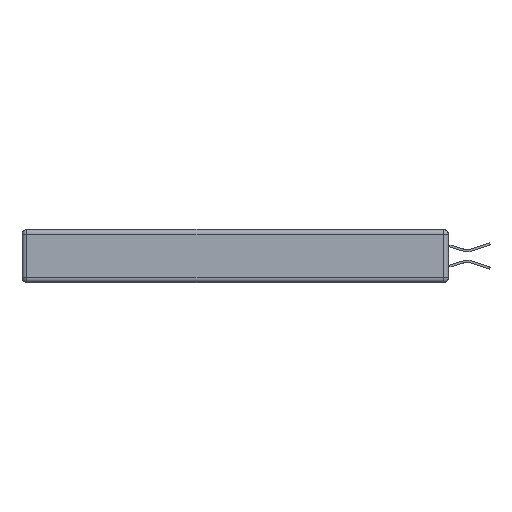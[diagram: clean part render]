
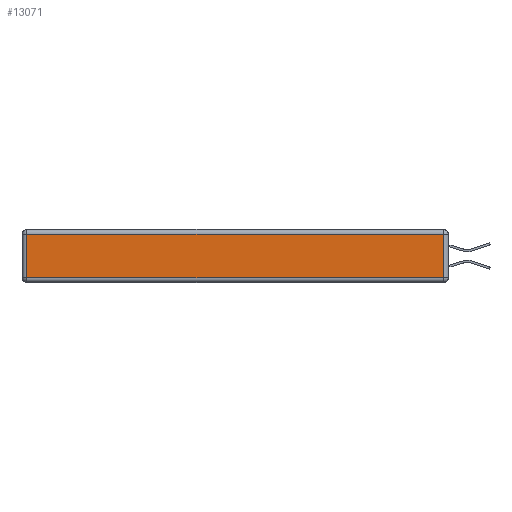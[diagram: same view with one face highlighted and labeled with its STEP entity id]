
A CAD part, left-side view. The second image highlights one B-rep face of the part: STEP entity #13071.
In plain terms, the highlighted planar face has unit normal (-1, 0, 0).
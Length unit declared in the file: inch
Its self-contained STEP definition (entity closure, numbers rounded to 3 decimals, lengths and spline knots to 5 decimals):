
#845 = CARTESIAN_POINT ( 'NONE',  ( 0., 2.72, -0.313 ) ) ;
#970 = VERTEX_POINT ( 'NONE', #845 ) ;
#1485 = EDGE_LOOP ( 'NONE', ( #31062, #12189, #10361, #12286 ) ) ;
#4456 = LINE ( 'NONE', #27313, #30382 ) ;
#4664 = CARTESIAN_POINT ( 'NONE',  ( 0., 0.03, -0.343 ) ) ;
#5438 = CARTESIAN_POINT ( 'NONE',  ( 0., 2.75, -0.03 ) ) ;
#6064 = LINE ( 'NONE', #5438, #15171 ) ;
#7155 = PLANE ( 'NONE',  #19806 ) ;
#8004 = DIRECTION ( 'NONE',  ( 0., 1., 0. ) ) ;
#8009 = CARTESIAN_POINT ( 'NONE',  ( 0., 0.03, -0.313 ) ) ;
#10361 = ORIENTED_EDGE ( 'NONE', *, *, #16900, .T. ) ;
#12189 = ORIENTED_EDGE ( 'NONE', *, *, #26618, .T. ) ;
#12286 = ORIENTED_EDGE ( 'NONE', *, *, #23566, .T. ) ;
#13071 = ADVANCED_FACE ( 'NONE', ( #21652 ), #7155, .T. ) ;
#14498 = VERTEX_POINT ( 'NONE', #23048 ) ;
#15023 = VERTEX_POINT ( 'NONE', #27066 ) ;
#15171 = VECTOR ( 'NONE', #8004, 39.37008 ) ;
#16363 = DIRECTION ( 'NONE',  ( 0., 0., 1. ) ) ;
#16900 = EDGE_CURVE ( 'NONE', #15023, #14498, #6064, .T. ) ;
#19366 = DIRECTION ( 'NONE',  ( -1., 0., 0. ) ) ;
#19806 = AXIS2_PLACEMENT_3D ( 'NONE', #31327, #19366, #24188 ) ;
#21652 = FACE_OUTER_BOUND ( 'NONE', #1485, .T. ) ;
#21655 = CARTESIAN_POINT ( 'NONE',  ( 0., 2.72, -0.343 ) ) ;
#22285 = DIRECTION ( 'NONE',  ( 0., -1., 0. ) ) ;
#23048 = CARTESIAN_POINT ( 'NONE',  ( 0., 2.72, -0.03 ) ) ;
#23566 = EDGE_CURVE ( 'NONE', #14498, #970, #24446, .T. ) ;
#24188 = DIRECTION ( 'NONE',  ( 0., 0., 1. ) ) ;
#24446 = LINE ( 'NONE', #21655, #29399 ) ;
#25673 = EDGE_CURVE ( 'NONE', #970, #28129, #4456, .T. ) ;
#26451 = DIRECTION ( 'NONE',  ( 0., 0., -1. ) ) ;
#26618 = EDGE_CURVE ( 'NONE', #28129, #15023, #27715, .T. ) ;
#27066 = CARTESIAN_POINT ( 'NONE',  ( 0., 0.03, -0.03 ) ) ;
#27313 = CARTESIAN_POINT ( 'NONE',  ( 0., 0., -0.313 ) ) ;
#27715 = LINE ( 'NONE', #4664, #28078 ) ;
#28078 = VECTOR ( 'NONE', #16363, 39.37008 ) ;
#28129 = VERTEX_POINT ( 'NONE', #8009 ) ;
#29399 = VECTOR ( 'NONE', #26451, 39.37008 ) ;
#30382 = VECTOR ( 'NONE', #22285, 39.37008 ) ;
#31062 = ORIENTED_EDGE ( 'NONE', *, *, #25673, .T. ) ;
#31327 = CARTESIAN_POINT ( 'NONE',  ( 0., 0., -0.343 ) ) ;
